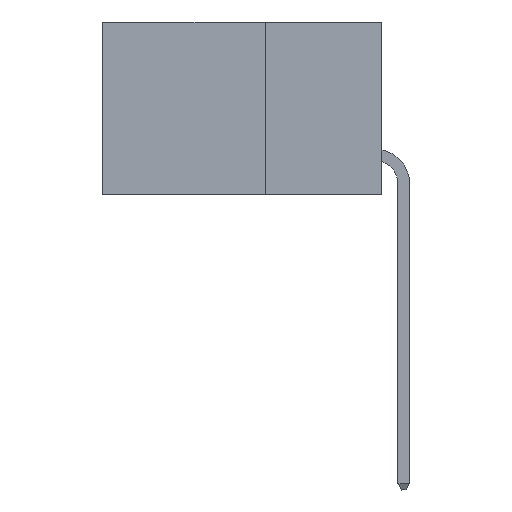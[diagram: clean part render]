
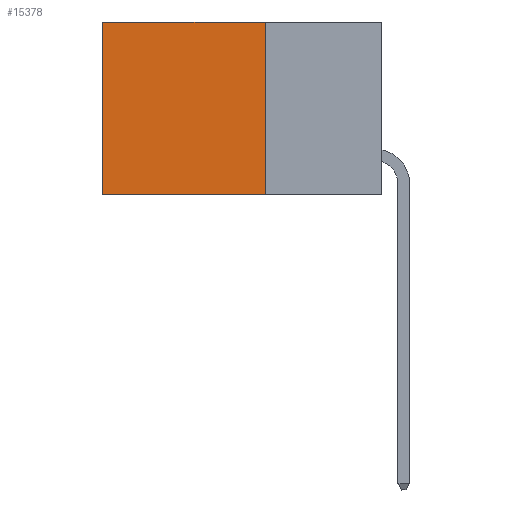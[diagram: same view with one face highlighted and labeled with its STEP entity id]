
A CAD part, left-side view. The second image highlights one B-rep face of the part: STEP entity #15378.
In plain terms, the highlighted planar face has unit normal (-1, 0, 0).
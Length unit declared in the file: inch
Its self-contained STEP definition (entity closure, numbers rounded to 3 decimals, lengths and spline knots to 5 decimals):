
#2352 = ORIENTED_EDGE ( 'NONE', *, *, #24374, .F. ) ;
#4013 = DIRECTION ( 'NONE',  ( 0., 0., -1. ) ) ;
#4086 = LINE ( 'NONE', #11169, #11161 ) ;
#4245 = EDGE_CURVE ( 'NONE', #24839, #28766, #4086, .T. ) ;
#9996 = VERTEX_POINT ( 'NONE', #30241 ) ;
#10190 = CARTESIAN_POINT ( 'NONE',  ( 0.2875, 0.25, -0.37 ) ) ;
#11161 = VECTOR ( 'NONE', #14406, 39.37008 ) ;
#11169 = CARTESIAN_POINT ( 'NONE',  ( 0.2875, 0.6, 0. ) ) ;
#11452 = CARTESIAN_POINT ( 'NONE',  ( 0.2875, 0.25, 0. ) ) ;
#12448 = CARTESIAN_POINT ( 'NONE',  ( 0.2875, 0.6, 0. ) ) ;
#13493 = ORIENTED_EDGE ( 'NONE', *, *, #4245, .T. ) ;
#14134 = FACE_OUTER_BOUND ( 'NONE', #29114, .T. ) ;
#14406 = DIRECTION ( 'NONE',  ( 0., 0., -1. ) ) ;
#15378 = ADVANCED_FACE ( 'NONE', ( #14134 ), #18374, .F. ) ;
#15986 = CARTESIAN_POINT ( 'NONE',  ( 0.2875, 0.25, 0. ) ) ;
#16344 = EDGE_CURVE ( 'NONE', #9996, #24839, #37005, .T. ) ;
#17826 = VECTOR ( 'NONE', #34366, 39.37008 ) ;
#18374 = PLANE ( 'NONE',  #24463 ) ;
#20141 = EDGE_CURVE ( 'NONE', #9996, #33858, #27457, .T. ) ;
#22315 = VECTOR ( 'NONE', #27015, 39.37008 ) ;
#22869 = DIRECTION ( 'NONE',  ( 0., 0., -1. ) ) ;
#23595 = VECTOR ( 'NONE', #22869, 39.37008 ) ;
#24374 = EDGE_CURVE ( 'NONE', #33858, #28766, #38600, .T. ) ;
#24463 = AXIS2_PLACEMENT_3D ( 'NONE', #11452, #32423, #4013 ) ;
#24839 = VERTEX_POINT ( 'NONE', #12448 ) ;
#27015 = DIRECTION ( 'NONE',  ( 0., 1., 0. ) ) ;
#27457 = LINE ( 'NONE', #15986, #23595 ) ;
#28766 = VERTEX_POINT ( 'NONE', #30257 ) ;
#29114 = EDGE_LOOP ( 'NONE', ( #13493, #2352, #39270, #42665 ) ) ;
#30241 = CARTESIAN_POINT ( 'NONE',  ( 0.2875, 0.25, 0. ) ) ;
#30257 = CARTESIAN_POINT ( 'NONE',  ( 0.2875, 0.6, -0.37 ) ) ;
#32423 = DIRECTION ( 'NONE',  ( 1., 0., 0. ) ) ;
#33858 = VERTEX_POINT ( 'NONE', #40886 ) ;
#34366 = DIRECTION ( 'NONE',  ( 0., 1., 0. ) ) ;
#37005 = LINE ( 'NONE', #37680, #22315 ) ;
#37680 = CARTESIAN_POINT ( 'NONE',  ( 0.2875, 0.25, 0. ) ) ;
#38600 = LINE ( 'NONE', #10190, #17826 ) ;
#39270 = ORIENTED_EDGE ( 'NONE', *, *, #20141, .F. ) ;
#40886 = CARTESIAN_POINT ( 'NONE',  ( 0.2875, 0.25, -0.37 ) ) ;
#42665 = ORIENTED_EDGE ( 'NONE', *, *, #16344, .T. ) ;
